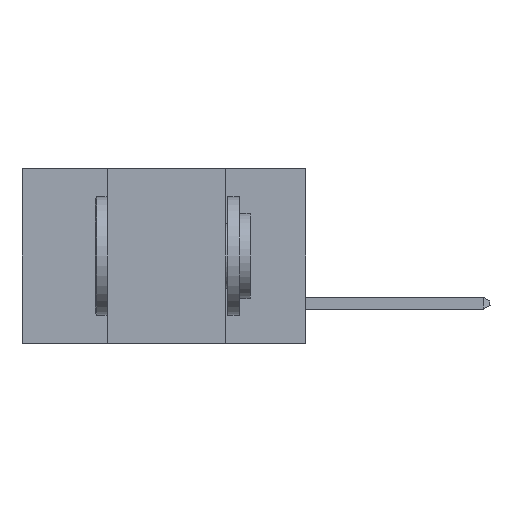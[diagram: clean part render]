
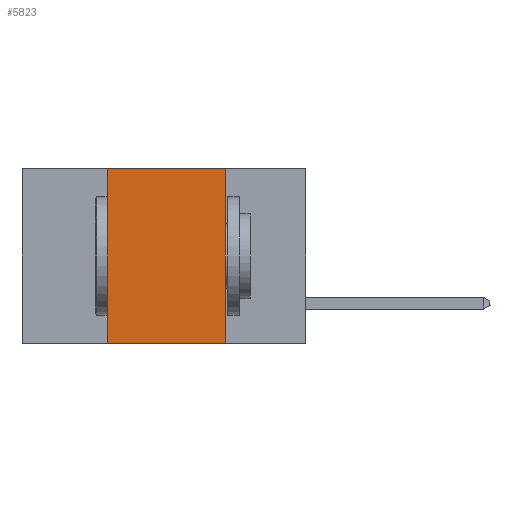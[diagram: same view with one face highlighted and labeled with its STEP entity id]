
A CAD part, left-side view. The second image highlights one B-rep face of the part: STEP entity #5823.
In plain terms, the highlighted planar face has unit normal (-1, 0, 0).
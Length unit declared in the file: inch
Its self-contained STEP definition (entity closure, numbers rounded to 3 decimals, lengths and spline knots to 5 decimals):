
#453 = LINE ( 'NONE', #15834, #4347 ) ;
#3238 = VECTOR ( 'NONE', #6652, 39.37008 ) ;
#3955 = ORIENTED_EDGE ( 'NONE', *, *, #12995, .F. ) ;
#4185 = ORIENTED_EDGE ( 'NONE', *, *, #12130, .F. ) ;
#4347 = VECTOR ( 'NONE', #17251, 39.37008 ) ;
#4511 = FACE_OUTER_BOUND ( 'NONE', #6226, .T. ) ;
#5088 = CARTESIAN_POINT ( 'NONE',  ( 0., 0.42, 0. ) ) ;
#5823 = ADVANCED_FACE ( 'NONE', ( #4511 ), #13606, .F. ) ;
#5837 = CARTESIAN_POINT ( 'NONE',  ( 0., 0.42, -0.37 ) ) ;
#6068 = CARTESIAN_POINT ( 'NONE',  ( 0., 0.42, 0. ) ) ;
#6069 = DIRECTION ( 'NONE',  ( 1., 0., 0. ) ) ;
#6226 = EDGE_LOOP ( 'NONE', ( #4185, #3955, #15840, #21365 ) ) ;
#6652 = DIRECTION ( 'NONE',  ( 0., 0., 1. ) ) ;
#6868 = CARTESIAN_POINT ( 'NONE',  ( 0., 0.6, 0. ) ) ;
#8683 = EDGE_CURVE ( 'NONE', #10947, #14047, #453, .T. ) ;
#9022 = VERTEX_POINT ( 'NONE', #13548 ) ;
#10227 = EDGE_CURVE ( 'NONE', #10947, #18245, #14650, .T. ) ;
#10303 = LINE ( 'NONE', #13335, #21052 ) ;
#10947 = VERTEX_POINT ( 'NONE', #5837 ) ;
#11053 = CARTESIAN_POINT ( 'NONE',  ( 0., 0.6, 0. ) ) ;
#12130 = EDGE_CURVE ( 'NONE', #9022, #14047, #10303, .T. ) ;
#12995 = EDGE_CURVE ( 'NONE', #18245, #9022, #19223, .T. ) ;
#13335 = CARTESIAN_POINT ( 'NONE',  ( 0., 0.17, 0. ) ) ;
#13548 = CARTESIAN_POINT ( 'NONE',  ( 0., 0.17, 0. ) ) ;
#13606 = PLANE ( 'NONE',  #19693 ) ;
#14047 = VERTEX_POINT ( 'NONE', #16064 ) ;
#14650 = LINE ( 'NONE', #5088, #3238 ) ;
#15501 = VECTOR ( 'NONE', #20453, 39.37008 ) ;
#15834 = CARTESIAN_POINT ( 'NONE',  ( 0., 0.6, -0.37 ) ) ;
#15840 = ORIENTED_EDGE ( 'NONE', *, *, #10227, .F. ) ;
#16064 = CARTESIAN_POINT ( 'NONE',  ( 0., 0.17, -0.37 ) ) ;
#17251 = DIRECTION ( 'NONE',  ( 0., -1., 0. ) ) ;
#18245 = VERTEX_POINT ( 'NONE', #6068 ) ;
#19223 = LINE ( 'NONE', #6868, #15501 ) ;
#19693 = AXIS2_PLACEMENT_3D ( 'NONE', #11053, #6069, #21017 ) ;
#20318 = DIRECTION ( 'NONE',  ( 0., 0., -1. ) ) ;
#20453 = DIRECTION ( 'NONE',  ( 0., -1., 0. ) ) ;
#21017 = DIRECTION ( 'NONE',  ( 0., 0., -1. ) ) ;
#21052 = VECTOR ( 'NONE', #20318, 39.37008 ) ;
#21365 = ORIENTED_EDGE ( 'NONE', *, *, #8683, .T. ) ;
